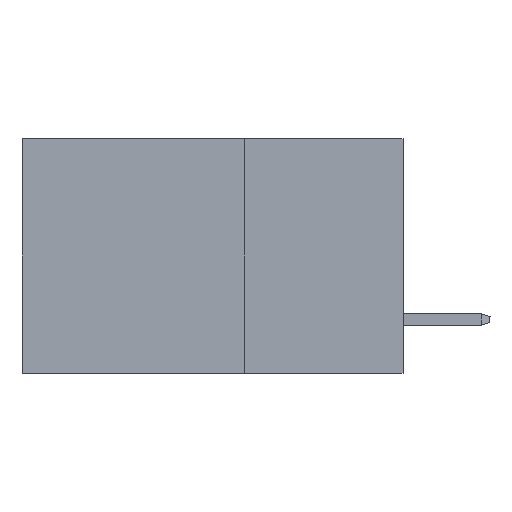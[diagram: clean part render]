
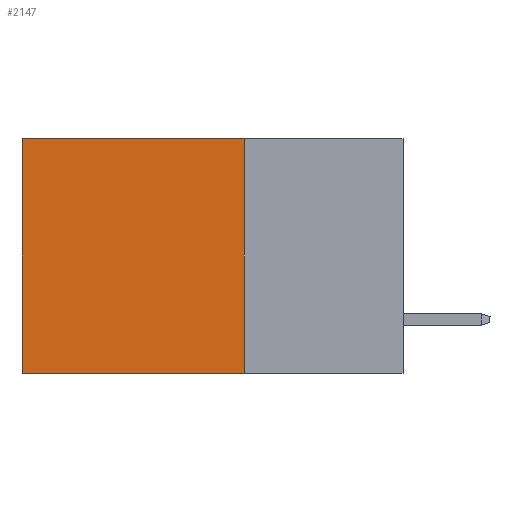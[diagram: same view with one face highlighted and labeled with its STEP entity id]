
A CAD part, left-side view. The second image highlights one B-rep face of the part: STEP entity #2147.
In plain terms, the highlighted planar face has unit normal (-1, 0, 0).
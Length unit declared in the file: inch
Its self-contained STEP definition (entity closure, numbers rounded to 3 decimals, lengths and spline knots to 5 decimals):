
#1622 = LINE ( 'NONE', #38640, #13107 ) ;
#1816 = CARTESIAN_POINT ( 'NONE',  ( 0.2875, 0.6, 0. ) ) ;
#2072 = VECTOR ( 'NONE', #17393, 39.37008 ) ;
#2147 = ADVANCED_FACE ( 'NONE', ( #26756 ), #10056, .F. ) ;
#2836 = ORIENTED_EDGE ( 'NONE', *, *, #22301, .F. ) ;
#3380 = CARTESIAN_POINT ( 'NONE',  ( 0.2875, 0.25, 0. ) ) ;
#4211 = CARTESIAN_POINT ( 'NONE',  ( 0.2875, 0.25, 0. ) ) ;
#5600 = CARTESIAN_POINT ( 'NONE',  ( 0.2875, 0.25, -0.37 ) ) ;
#7251 = EDGE_CURVE ( 'NONE', #36641, #19509, #38455, .T. ) ;
#7602 = ORIENTED_EDGE ( 'NONE', *, *, #41591, .F. ) ;
#9834 = DIRECTION ( 'NONE',  ( 0., 0., -1. ) ) ;
#10029 = VERTEX_POINT ( 'NONE', #14791 ) ;
#10056 = PLANE ( 'NONE',  #29828 ) ;
#12528 = DIRECTION ( 'NONE',  ( 0., 1., 0. ) ) ;
#13107 = VECTOR ( 'NONE', #15026, 39.37008 ) ;
#14791 = CARTESIAN_POINT ( 'NONE',  ( 0.2875, 0.25, 0. ) ) ;
#15026 = DIRECTION ( 'NONE',  ( 0., 0., -1. ) ) ;
#15837 = CARTESIAN_POINT ( 'NONE',  ( 0.2875, 0.6, -0.37 ) ) ;
#16782 = VECTOR ( 'NONE', #26070, 39.37008 ) ;
#17393 = DIRECTION ( 'NONE',  ( 0., 1., 0. ) ) ;
#17668 = ORIENTED_EDGE ( 'NONE', *, *, #41523, .T. ) ;
#19130 = CARTESIAN_POINT ( 'NONE',  ( 0.2875, 0.25, -0.37 ) ) ;
#19509 = VERTEX_POINT ( 'NONE', #15837 ) ;
#20838 = LINE ( 'NONE', #4211, #2072 ) ;
#22301 = EDGE_CURVE ( 'NONE', #28355, #19509, #35301, .T. ) ;
#26070 = DIRECTION ( 'NONE',  ( 0., 0., -1. ) ) ;
#26756 = FACE_OUTER_BOUND ( 'NONE', #38607, .T. ) ;
#28355 = VERTEX_POINT ( 'NONE', #19130 ) ;
#29828 = AXIS2_PLACEMENT_3D ( 'NONE', #3380, #39543, #9834 ) ;
#31345 = ORIENTED_EDGE ( 'NONE', *, *, #7251, .T. ) ;
#33565 = VECTOR ( 'NONE', #12528, 39.37008 ) ;
#35301 = LINE ( 'NONE', #5600, #33565 ) ;
#35844 = CARTESIAN_POINT ( 'NONE',  ( 0.2875, 0.6, 0. ) ) ;
#36641 = VERTEX_POINT ( 'NONE', #1816 ) ;
#38455 = LINE ( 'NONE', #35844, #16782 ) ;
#38607 = EDGE_LOOP ( 'NONE', ( #31345, #2836, #7602, #17668 ) ) ;
#38640 = CARTESIAN_POINT ( 'NONE',  ( 0.2875, 0.25, 0. ) ) ;
#39543 = DIRECTION ( 'NONE',  ( 1., 0., 0. ) ) ;
#41523 = EDGE_CURVE ( 'NONE', #10029, #36641, #20838, .T. ) ;
#41591 = EDGE_CURVE ( 'NONE', #10029, #28355, #1622, .T. ) ;
